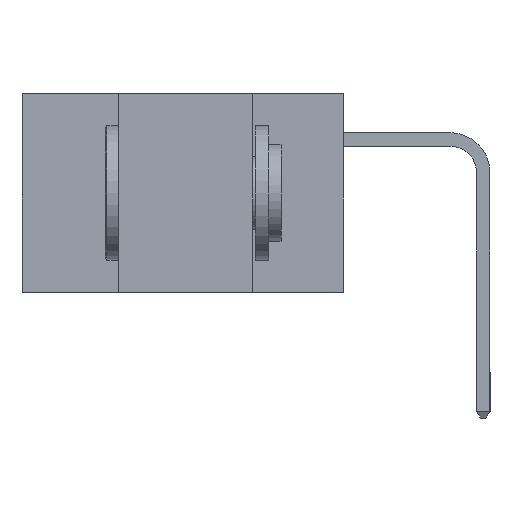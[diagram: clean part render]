
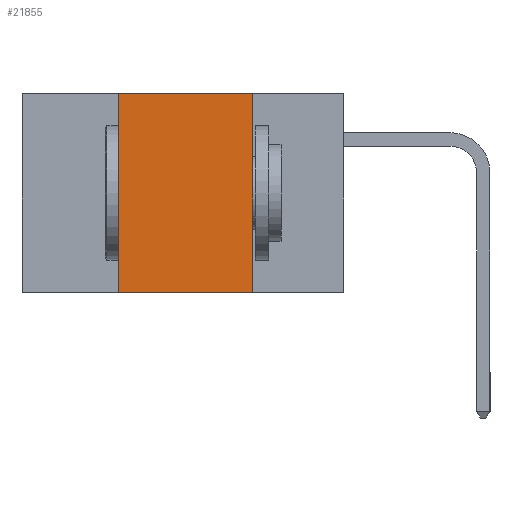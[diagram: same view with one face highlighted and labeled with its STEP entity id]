
A CAD part, left-side view. The second image highlights one B-rep face of the part: STEP entity #21855.
In plain terms, the highlighted planar face has unit normal (-1, 0, 0).
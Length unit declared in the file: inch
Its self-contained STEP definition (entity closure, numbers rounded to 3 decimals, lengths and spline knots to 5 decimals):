
#1205 = CARTESIAN_POINT ( 'NONE',  ( 0., 0.17, 0. ) ) ;
#1489 = DIRECTION ( 'NONE',  ( 0., -1., 0. ) ) ;
#2921 = VERTEX_POINT ( 'NONE', #8801 ) ;
#4077 = ORIENTED_EDGE ( 'NONE', *, *, #19973, .T. ) ;
#4610 = VECTOR ( 'NONE', #24961, 39.37008 ) ;
#6501 = CARTESIAN_POINT ( 'NONE',  ( 0., 0.42, 0. ) ) ;
#7350 = CARTESIAN_POINT ( 'NONE',  ( 0., 0.6, -0.37 ) ) ;
#7538 = DIRECTION ( 'NONE',  ( 0., 0., -1. ) ) ;
#8756 = FACE_OUTER_BOUND ( 'NONE', #21725, .T. ) ;
#8801 = CARTESIAN_POINT ( 'NONE',  ( 0., 0.42, -0.37 ) ) ;
#9414 = LINE ( 'NONE', #7350, #20258 ) ;
#10518 = VERTEX_POINT ( 'NONE', #12680 ) ;
#10884 = CARTESIAN_POINT ( 'NONE',  ( 0., 0.6, 0. ) ) ;
#10963 = PLANE ( 'NONE',  #18011 ) ;
#11191 = VERTEX_POINT ( 'NONE', #14709 ) ;
#11544 = DIRECTION ( 'NONE',  ( 0., -1., 0. ) ) ;
#11652 = EDGE_CURVE ( 'NONE', #11191, #14956, #13399, .T. ) ;
#11663 = LINE ( 'NONE', #6501, #4610 ) ;
#12680 = CARTESIAN_POINT ( 'NONE',  ( 0., 0.17, -0.37 ) ) ;
#13399 = LINE ( 'NONE', #15628, #16611 ) ;
#14709 = CARTESIAN_POINT ( 'NONE',  ( 0., 0.42, 0. ) ) ;
#14739 = DIRECTION ( 'NONE',  ( 1., 0., 0. ) ) ;
#14956 = VERTEX_POINT ( 'NONE', #1205 ) ;
#15628 = CARTESIAN_POINT ( 'NONE',  ( 0., 0.6, 0. ) ) ;
#16611 = VECTOR ( 'NONE', #1489, 39.37008 ) ;
#17028 = EDGE_CURVE ( 'NONE', #2921, #11191, #11663, .T. ) ;
#17235 = ORIENTED_EDGE ( 'NONE', *, *, #17028, .F. ) ;
#17622 = CARTESIAN_POINT ( 'NONE',  ( 0., 0.17, 0. ) ) ;
#17676 = VECTOR ( 'NONE', #7538, 39.37008 ) ;
#18011 = AXIS2_PLACEMENT_3D ( 'NONE', #10884, #14739, #23222 ) ;
#19637 = ORIENTED_EDGE ( 'NONE', *, *, #23427, .F. ) ;
#19973 = EDGE_CURVE ( 'NONE', #2921, #10518, #9414, .T. ) ;
#20258 = VECTOR ( 'NONE', #11544, 39.37008 ) ;
#21725 = EDGE_LOOP ( 'NONE', ( #19637, #24898, #17235, #4077 ) ) ;
#21855 = ADVANCED_FACE ( 'NONE', ( #8756 ), #10963, .F. ) ;
#23129 = LINE ( 'NONE', #17622, #17676 ) ;
#23222 = DIRECTION ( 'NONE',  ( 0., 0., -1. ) ) ;
#23427 = EDGE_CURVE ( 'NONE', #14956, #10518, #23129, .T. ) ;
#24898 = ORIENTED_EDGE ( 'NONE', *, *, #11652, .F. ) ;
#24961 = DIRECTION ( 'NONE',  ( 0., 0., 1. ) ) ;
